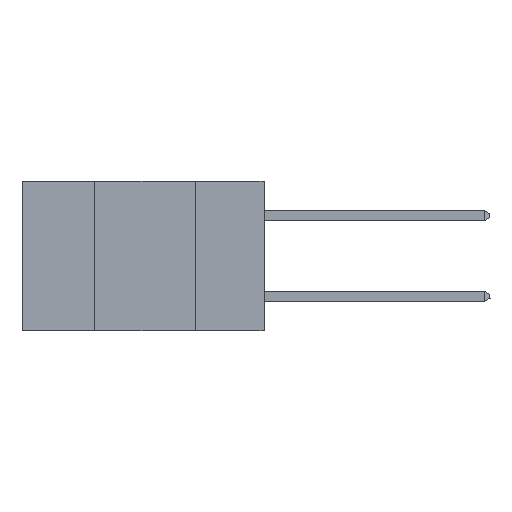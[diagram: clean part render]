
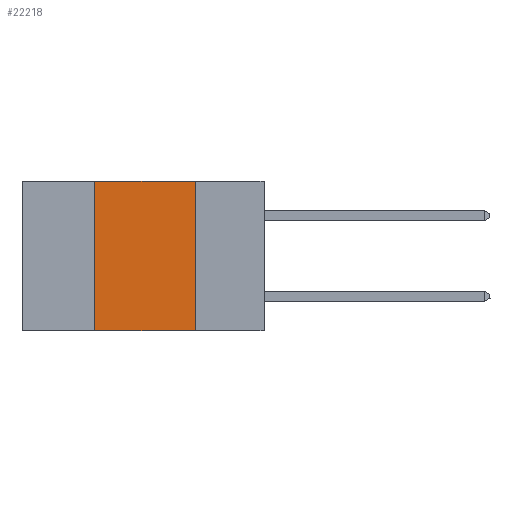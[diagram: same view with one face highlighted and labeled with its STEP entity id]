
A CAD part, left-side view. The second image highlights one B-rep face of the part: STEP entity #22218.
In plain terms, the highlighted planar face has unit normal (-1, 0, 0).
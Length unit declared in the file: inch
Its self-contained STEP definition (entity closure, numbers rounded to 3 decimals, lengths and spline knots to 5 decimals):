
#65 = DIRECTION ( 'NONE',  ( 1., 0., 0. ) ) ;
#1100 = VERTEX_POINT ( 'NONE', #27374 ) ;
#1784 = CARTESIAN_POINT ( 'NONE',  ( 0., 0.42, -0.37 ) ) ;
#2565 = FACE_OUTER_BOUND ( 'NONE', #12692, .T. ) ;
#3063 = ORIENTED_EDGE ( 'NONE', *, *, #15962, .F. ) ;
#3636 = LINE ( 'NONE', #16226, #4326 ) ;
#4326 = VECTOR ( 'NONE', #24686, 39.37008 ) ;
#5470 = VERTEX_POINT ( 'NONE', #21528 ) ;
#8947 = CARTESIAN_POINT ( 'NONE',  ( 0., 0.6, 0. ) ) ;
#9504 = VECTOR ( 'NONE', #13804, 39.37008 ) ;
#9750 = VERTEX_POINT ( 'NONE', #27493 ) ;
#9773 = VERTEX_POINT ( 'NONE', #17520 ) ;
#10866 = VECTOR ( 'NONE', #21754, 39.37008 ) ;
#11729 = ORIENTED_EDGE ( 'NONE', *, *, #20617, .F. ) ;
#12692 = EDGE_LOOP ( 'NONE', ( #23115, #3063, #11729, #18837 ) ) ;
#12986 = CARTESIAN_POINT ( 'NONE',  ( 0., 0.6, 0. ) ) ;
#13804 = DIRECTION ( 'NONE',  ( 0., 0., -1. ) ) ;
#14668 = DIRECTION ( 'NONE',  ( 0., 0., 1. ) ) ;
#15161 = DIRECTION ( 'NONE',  ( 0., 0., -1. ) ) ;
#15962 = EDGE_CURVE ( 'NONE', #9750, #1100, #22250, .T. ) ;
#16226 = CARTESIAN_POINT ( 'NONE',  ( 0., 0.6, -0.37 ) ) ;
#17520 = CARTESIAN_POINT ( 'NONE',  ( 0., 0.42, -0.37 ) ) ;
#18829 = EDGE_CURVE ( 'NONE', #1100, #5470, #21547, .T. ) ;
#18837 = ORIENTED_EDGE ( 'NONE', *, *, #26807, .T. ) ;
#20055 = AXIS2_PLACEMENT_3D ( 'NONE', #12986, #65, #15161 ) ;
#20617 = EDGE_CURVE ( 'NONE', #9773, #9750, #26753, .T. ) ;
#21146 = VECTOR ( 'NONE', #14668, 39.37008 ) ;
#21528 = CARTESIAN_POINT ( 'NONE',  ( 0., 0.17, -0.37 ) ) ;
#21547 = LINE ( 'NONE', #26545, #9504 ) ;
#21754 = DIRECTION ( 'NONE',  ( 0., -1., 0. ) ) ;
#22218 = ADVANCED_FACE ( 'NONE', ( #2565 ), #23620, .F. ) ;
#22250 = LINE ( 'NONE', #8947, #10866 ) ;
#23115 = ORIENTED_EDGE ( 'NONE', *, *, #18829, .F. ) ;
#23620 = PLANE ( 'NONE',  #20055 ) ;
#24686 = DIRECTION ( 'NONE',  ( 0., -1., 0. ) ) ;
#26545 = CARTESIAN_POINT ( 'NONE',  ( 0., 0.17, -0.37 ) ) ;
#26753 = LINE ( 'NONE', #1784, #21146 ) ;
#26807 = EDGE_CURVE ( 'NONE', #9773, #5470, #3636, .T. ) ;
#27374 = CARTESIAN_POINT ( 'NONE',  ( 0., 0.17, 0. ) ) ;
#27493 = CARTESIAN_POINT ( 'NONE',  ( 0., 0.42, 0. ) ) ;
